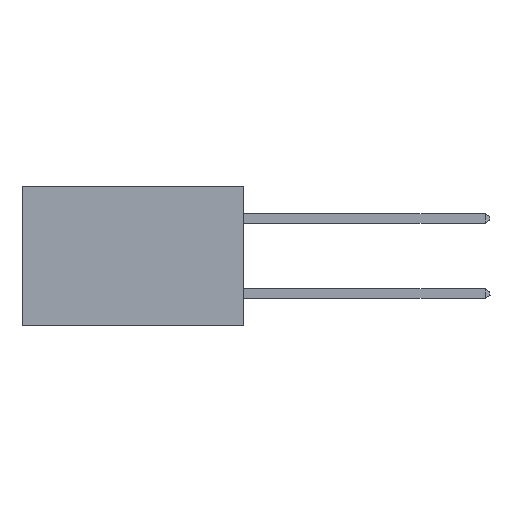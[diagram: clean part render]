
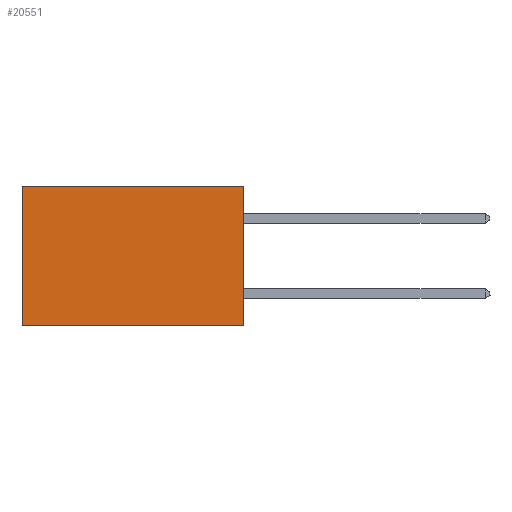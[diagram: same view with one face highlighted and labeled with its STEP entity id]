
A CAD part, left-side view. The second image highlights one B-rep face of the part: STEP entity #20551.
In plain terms, the highlighted planar face has unit normal (-1, 0, 0).
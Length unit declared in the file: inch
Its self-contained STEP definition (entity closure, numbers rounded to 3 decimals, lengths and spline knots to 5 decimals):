
#445 = ORIENTED_EDGE ( 'NONE', *, *, #25986, .F. ) ;
#1157 = ORIENTED_EDGE ( 'NONE', *, *, #21913, .F. ) ;
#2927 = CARTESIAN_POINT ( 'NONE',  ( 0.277, 0., 0. ) ) ;
#3192 = CARTESIAN_POINT ( 'NONE',  ( 0.277, 0.59, -0.37 ) ) ;
#7550 = DIRECTION ( 'NONE',  ( 1., 0., 0. ) ) ;
#7709 = CARTESIAN_POINT ( 'NONE',  ( 0.277, 0.59, -0.37 ) ) ;
#7814 = ORIENTED_EDGE ( 'NONE', *, *, #13249, .T. ) ;
#8086 = EDGE_LOOP ( 'NONE', ( #19224, #445, #1157, #7814 ) ) ;
#8136 = VECTOR ( 'NONE', #25149, 39.37008 ) ;
#8747 = LINE ( 'NONE', #20879, #25102 ) ;
#8752 = AXIS2_PLACEMENT_3D ( 'NONE', #14149, #7550, #23118 ) ;
#8830 = LINE ( 'NONE', #14070, #8136 ) ;
#8909 = FACE_OUTER_BOUND ( 'NONE', #8086, .T. ) ;
#10694 = CARTESIAN_POINT ( 'NONE',  ( 0.277, 0., 0. ) ) ;
#11002 = CARTESIAN_POINT ( 'NONE',  ( 0.277, 0.59, 0. ) ) ;
#11982 = DIRECTION ( 'NONE',  ( 0., 1., 0. ) ) ;
#12923 = DIRECTION ( 'NONE',  ( 0., 1., 0. ) ) ;
#13249 = EDGE_CURVE ( 'NONE', #13630, #20924, #28182, .T. ) ;
#13630 = VERTEX_POINT ( 'NONE', #2927 ) ;
#14070 = CARTESIAN_POINT ( 'NONE',  ( 0.277, 0., -0.37 ) ) ;
#14149 = CARTESIAN_POINT ( 'NONE',  ( 0.277, 0., -0.37 ) ) ;
#15156 = VERTEX_POINT ( 'NONE', #7709 ) ;
#17926 = CARTESIAN_POINT ( 'NONE',  ( 0.277, 0., -0.37 ) ) ;
#18667 = PLANE ( 'NONE',  #8752 ) ;
#19224 = ORIENTED_EDGE ( 'NONE', *, *, #19872, .T. ) ;
#19872 = EDGE_CURVE ( 'NONE', #20924, #15156, #26606, .T. ) ;
#20551 = ADVANCED_FACE ( 'NONE', ( #8909 ), #18667, .F. ) ;
#20879 = CARTESIAN_POINT ( 'NONE',  ( 0.277, 0., -0.37 ) ) ;
#20924 = VERTEX_POINT ( 'NONE', #11002 ) ;
#21048 = DIRECTION ( 'NONE',  ( 0., 0., -1. ) ) ;
#21913 = EDGE_CURVE ( 'NONE', #13630, #28431, #8830, .T. ) ;
#22415 = VECTOR ( 'NONE', #12923, 39.37008 ) ;
#23118 = DIRECTION ( 'NONE',  ( 0., 0., -1. ) ) ;
#25102 = VECTOR ( 'NONE', #11982, 39.37008 ) ;
#25149 = DIRECTION ( 'NONE',  ( 0., 0., -1. ) ) ;
#25986 = EDGE_CURVE ( 'NONE', #28431, #15156, #8747, .T. ) ;
#26606 = LINE ( 'NONE', #3192, #27298 ) ;
#27298 = VECTOR ( 'NONE', #21048, 39.37008 ) ;
#28182 = LINE ( 'NONE', #10694, #22415 ) ;
#28431 = VERTEX_POINT ( 'NONE', #17926 ) ;
